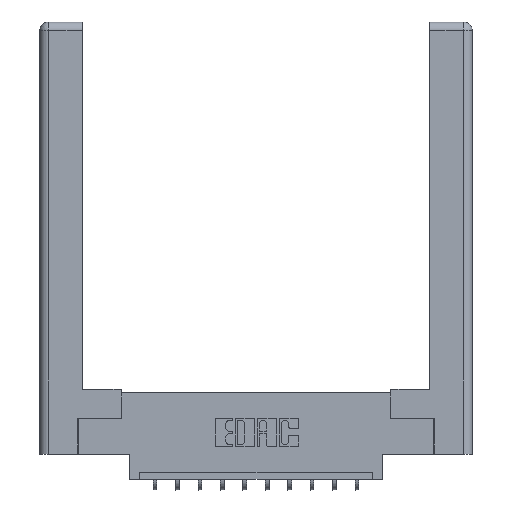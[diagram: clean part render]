
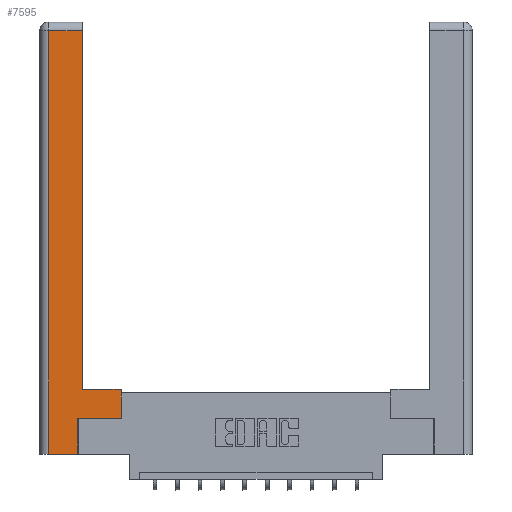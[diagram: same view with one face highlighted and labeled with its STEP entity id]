
A CAD part, top view. The second image highlights one B-rep face of the part: STEP entity #7595.
In plain terms, the highlighted planar face has unit normal (0, 0, 1).
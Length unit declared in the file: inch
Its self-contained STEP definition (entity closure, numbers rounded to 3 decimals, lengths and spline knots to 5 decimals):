
#38 = VERTEX_POINT ( 'NONE', #13384 ) ;
#81 = DIRECTION ( 'NONE',  ( -1., 0., 0. ) ) ;
#477 = DIRECTION ( 'NONE',  ( 1., 0., 0. ) ) ;
#1366 = CARTESIAN_POINT ( 'NONE',  ( 0.0615, 0., 0. ) ) ;
#1446 = LINE ( 'NONE', #9302, #11212 ) ;
#2104 = DIRECTION ( 'NONE',  ( -1., 0., 0. ) ) ;
#2138 = CARTESIAN_POINT ( 'NONE',  ( 0.0615, 0., 0. ) ) ;
#2184 = DIRECTION ( 'NONE',  ( 0., -1., 0. ) ) ;
#2552 = ORIENTED_EDGE ( 'NONE', *, *, #11820, .T. ) ;
#3282 = LINE ( 'NONE', #12394, #5727 ) ;
#3323 = VECTOR ( 'NONE', #7229, 39.37008 ) ;
#3629 = ORIENTED_EDGE ( 'NONE', *, *, #12647, .T. ) ;
#3739 = EDGE_CURVE ( 'NONE', #7084, #6445, #7842, .T. ) ;
#4310 = DIRECTION ( 'NONE',  ( 0., 1., 0. ) ) ;
#4359 = VERTEX_POINT ( 'NONE', #5617 ) ;
#4541 = LINE ( 'NONE', #8852, #12420 ) ;
#4964 = VECTOR ( 'NONE', #14072, 39.37008 ) ;
#5311 = LINE ( 'NONE', #14262, #4964 ) ;
#5365 = LINE ( 'NONE', #9881, #13958 ) ;
#5457 = CARTESIAN_POINT ( 'NONE',  ( 0.265, 0.245, 0. ) ) ;
#5465 = VECTOR ( 'NONE', #2184, 39.37008 ) ;
#5543 = VERTEX_POINT ( 'NONE', #5457 ) ;
#5617 = CARTESIAN_POINT ( 'NONE',  ( 0.295, 0.45, 0. ) ) ;
#5727 = VECTOR ( 'NONE', #7986, 39.37008 ) ;
#6055 = ORIENTED_EDGE ( 'NONE', *, *, #3739, .T. ) ;
#6099 = CARTESIAN_POINT ( 'NONE',  ( 0.295, 2.94, 0. ) ) ;
#6180 = ORIENTED_EDGE ( 'NONE', *, *, #9308, .T. ) ;
#6349 = AXIS2_PLACEMENT_3D ( 'NONE', #12123, #10259, #13631 ) ;
#6414 = VERTEX_POINT ( 'NONE', #1366 ) ;
#6445 = VERTEX_POINT ( 'NONE', #6752 ) ;
#6752 = CARTESIAN_POINT ( 'NONE',  ( 0.0615, 2.94, 0. ) ) ;
#7084 = VERTEX_POINT ( 'NONE', #6099 ) ;
#7229 = DIRECTION ( 'NONE',  ( 0., 1., 0. ) ) ;
#7595 = ADVANCED_FACE ( 'NONE', ( #11423 ), #9853, .F. ) ;
#7607 = EDGE_CURVE ( 'NONE', #6445, #6414, #10900, .T. ) ;
#7842 = LINE ( 'NONE', #13378, #13460 ) ;
#7986 = DIRECTION ( 'NONE',  ( 1., 0., 0. ) ) ;
#8314 = CARTESIAN_POINT ( 'NONE',  ( 0.265, 0.245, 0. ) ) ;
#8852 = CARTESIAN_POINT ( 'NONE',  ( 0.295, 0.45, 0. ) ) ;
#9287 = ORIENTED_EDGE ( 'NONE', *, *, #13129, .T. ) ;
#9302 = CARTESIAN_POINT ( 'NONE',  ( 0.265, 0., 0. ) ) ;
#9308 = EDGE_CURVE ( 'NONE', #4359, #7084, #5311, .T. ) ;
#9853 = PLANE ( 'NONE',  #6349 ) ;
#9881 = CARTESIAN_POINT ( 'NONE',  ( 0.565, 0.45, 0. ) ) ;
#10235 = ORIENTED_EDGE ( 'NONE', *, *, #11084, .T. ) ;
#10259 = DIRECTION ( 'NONE',  ( 0., 0., -1. ) ) ;
#10565 = CARTESIAN_POINT ( 'NONE',  ( 0.565, 0.45, 0. ) ) ;
#10688 = EDGE_LOOP ( 'NONE', ( #6180, #6055, #13265, #10235, #11394, #3629, #9287, #2552 ) ) ;
#10900 = LINE ( 'NONE', #2138, #5465 ) ;
#11084 = EDGE_CURVE ( 'NONE', #6414, #13695, #1446, .T. ) ;
#11212 = VECTOR ( 'NONE', #477, 39.37008 ) ;
#11394 = ORIENTED_EDGE ( 'NONE', *, *, #11522, .T. ) ;
#11423 = FACE_OUTER_BOUND ( 'NONE', #10688, .T. ) ;
#11522 = EDGE_CURVE ( 'NONE', #13695, #5543, #12253, .T. ) ;
#11747 = CARTESIAN_POINT ( 'NONE',  ( 0.265, 0., 0. ) ) ;
#11820 = EDGE_CURVE ( 'NONE', #13439, #4359, #4541, .T. ) ;
#12123 = CARTESIAN_POINT ( 'NONE',  ( 0., 0., 0. ) ) ;
#12253 = LINE ( 'NONE', #8314, #3323 ) ;
#12394 = CARTESIAN_POINT ( 'NONE',  ( 0.565, 0.245, 0. ) ) ;
#12420 = VECTOR ( 'NONE', #2104, 39.37008 ) ;
#12647 = EDGE_CURVE ( 'NONE', #5543, #38, #3282, .T. ) ;
#13129 = EDGE_CURVE ( 'NONE', #38, #13439, #5365, .T. ) ;
#13265 = ORIENTED_EDGE ( 'NONE', *, *, #7607, .T. ) ;
#13378 = CARTESIAN_POINT ( 'NONE',  ( 0.0615, 2.94, 0. ) ) ;
#13384 = CARTESIAN_POINT ( 'NONE',  ( 0.565, 0.245, 0. ) ) ;
#13439 = VERTEX_POINT ( 'NONE', #10565 ) ;
#13460 = VECTOR ( 'NONE', #81, 39.37008 ) ;
#13631 = DIRECTION ( 'NONE',  ( -1., 0., 0. ) ) ;
#13695 = VERTEX_POINT ( 'NONE', #11747 ) ;
#13958 = VECTOR ( 'NONE', #4310, 39.37008 ) ;
#14072 = DIRECTION ( 'NONE',  ( 0., 1., 0. ) ) ;
#14262 = CARTESIAN_POINT ( 'NONE',  ( 0.295, 3., 0. ) ) ;
